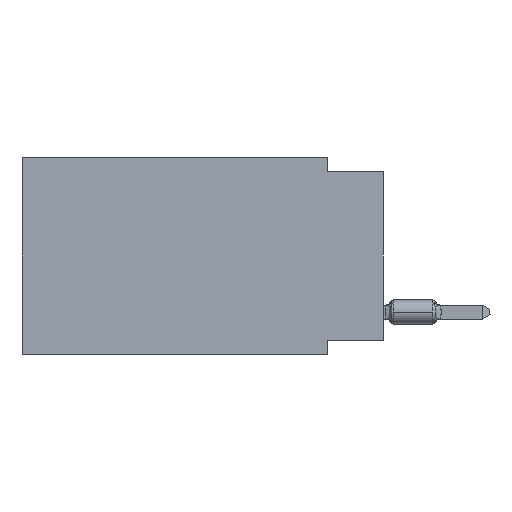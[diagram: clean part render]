
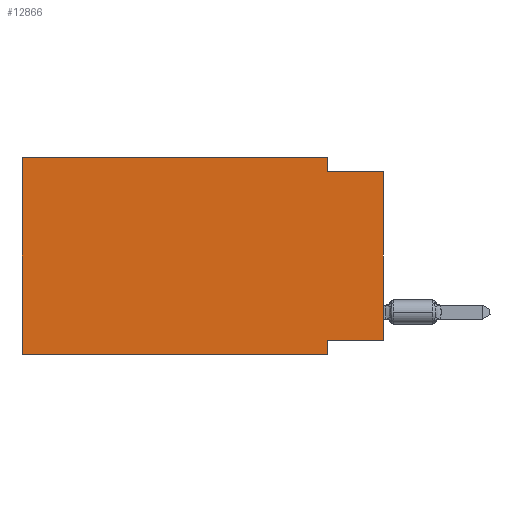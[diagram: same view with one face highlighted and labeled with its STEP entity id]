
A CAD part, left-side view. The second image highlights one B-rep face of the part: STEP entity #12866.
In plain terms, the highlighted planar face has unit normal (-1, 0, 0).
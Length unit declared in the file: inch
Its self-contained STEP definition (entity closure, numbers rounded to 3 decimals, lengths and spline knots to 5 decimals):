
#143 = EDGE_LOOP ( 'NONE', ( #57750, #5036, #26587, #40069, #41600, #67561, #18954, #63078 ) ) ;
#573 = LINE ( 'NONE', #1650, #47696 ) ;
#854 = CARTESIAN_POINT ( 'NONE',  ( 0., 0., -0.025 ) ) ;
#1492 = DIRECTION ( 'NONE',  ( 0., -1., 0. ) ) ;
#1650 = CARTESIAN_POINT ( 'NONE',  ( 0., 0., 0. ) ) ;
#2251 = VERTEX_POINT ( 'NONE', #854 ) ;
#2700 = AXIS2_PLACEMENT_3D ( 'NONE', #33103, #27999, #16654 ) ;
#3034 = EDGE_CURVE ( 'NONE', #63073, #41070, #44069, .T. ) ;
#5036 = ORIENTED_EDGE ( 'NONE', *, *, #12975, .F. ) ;
#5230 = EDGE_CURVE ( 'NONE', #29699, #2251, #573, .T. ) ;
#5494 = VERTEX_POINT ( 'NONE', #10653 ) ;
#9241 = VERTEX_POINT ( 'NONE', #39846 ) ;
#10653 = CARTESIAN_POINT ( 'NONE',  ( 0., 0.1, 0. ) ) ;
#12866 = ADVANCED_FACE ( 'NONE', ( #37851 ), #61591, .F. ) ;
#12975 = EDGE_CURVE ( 'NONE', #13869, #2251, #32755, .T. ) ;
#13869 = VERTEX_POINT ( 'NONE', #43752 ) ;
#14903 = VECTOR ( 'NONE', #70782, 39.37008 ) ;
#15004 = LINE ( 'NONE', #15367, #36095 ) ;
#15367 = CARTESIAN_POINT ( 'NONE',  ( 0., 0., -0.325 ) ) ;
#16654 = DIRECTION ( 'NONE',  ( 0., 0., -1. ) ) ;
#17293 = CARTESIAN_POINT ( 'NONE',  ( 0., 0.645, -0.35 ) ) ;
#18954 = ORIENTED_EDGE ( 'NONE', *, *, #43424, .F. ) ;
#20109 = LINE ( 'NONE', #42380, #58778 ) ;
#21126 = CARTESIAN_POINT ( 'NONE',  ( 0., 0.1, -0.35 ) ) ;
#21906 = CARTESIAN_POINT ( 'NONE',  ( 0., 0.1, -0.35 ) ) ;
#22706 = CARTESIAN_POINT ( 'NONE',  ( 0., 0.645, -0.35 ) ) ;
#26019 = VECTOR ( 'NONE', #44044, 39.37008 ) ;
#26307 = DIRECTION ( 'NONE',  ( 0., -1., 0. ) ) ;
#26587 = ORIENTED_EDGE ( 'NONE', *, *, #45945, .F. ) ;
#26660 = EDGE_CURVE ( 'NONE', #41070, #5494, #20109, .T. ) ;
#27999 = DIRECTION ( 'NONE',  ( 1., 0., 0. ) ) ;
#28007 = DIRECTION ( 'NONE',  ( 0., 0., 1. ) ) ;
#29699 = VERTEX_POINT ( 'NONE', #39610 ) ;
#32711 = EDGE_CURVE ( 'NONE', #29699, #9241, #15004, .T. ) ;
#32755 = LINE ( 'NONE', #55020, #26019 ) ;
#33103 = CARTESIAN_POINT ( 'NONE',  ( 0., 0.645, 0. ) ) ;
#33259 = DIRECTION ( 'NONE',  ( 0., 0., -1. ) ) ;
#36095 = VECTOR ( 'NONE', #47892, 39.37008 ) ;
#37851 = FACE_OUTER_BOUND ( 'NONE', #143, .T. ) ;
#39610 = CARTESIAN_POINT ( 'NONE',  ( 0., 0., -0.325 ) ) ;
#39846 = CARTESIAN_POINT ( 'NONE',  ( 0., 0.1, -0.325 ) ) ;
#40069 = ORIENTED_EDGE ( 'NONE', *, *, #26660, .F. ) ;
#40533 = LINE ( 'NONE', #62452, #57853 ) ;
#41070 = VERTEX_POINT ( 'NONE', #47830 ) ;
#41600 = ORIENTED_EDGE ( 'NONE', *, *, #3034, .F. ) ;
#42380 = CARTESIAN_POINT ( 'NONE',  ( 0., 0.645, 0. ) ) ;
#43424 = EDGE_CURVE ( 'NONE', #9241, #46297, #48925, .T. ) ;
#43752 = CARTESIAN_POINT ( 'NONE',  ( 0., 0.1, -0.025 ) ) ;
#43954 = VECTOR ( 'NONE', #1492, 39.37008 ) ;
#44044 = DIRECTION ( 'NONE',  ( 0., -1., 0. ) ) ;
#44069 = LINE ( 'NONE', #60894, #14903 ) ;
#44167 = DIRECTION ( 'NONE',  ( 0., 0., -1. ) ) ;
#45945 = EDGE_CURVE ( 'NONE', #5494, #13869, #40533, .T. ) ;
#46297 = VERTEX_POINT ( 'NONE', #21126 ) ;
#47696 = VECTOR ( 'NONE', #28007, 39.37008 ) ;
#47830 = CARTESIAN_POINT ( 'NONE',  ( 0., 0.645, 0. ) ) ;
#47892 = DIRECTION ( 'NONE',  ( 0., 1., 0. ) ) ;
#48925 = LINE ( 'NONE', #21906, #71616 ) ;
#51552 = LINE ( 'NONE', #22706, #43954 ) ;
#55020 = CARTESIAN_POINT ( 'NONE',  ( 0., 0., -0.025 ) ) ;
#57750 = ORIENTED_EDGE ( 'NONE', *, *, #5230, .T. ) ;
#57853 = VECTOR ( 'NONE', #33259, 39.37008 ) ;
#58778 = VECTOR ( 'NONE', #26307, 39.37008 ) ;
#60894 = CARTESIAN_POINT ( 'NONE',  ( 0., 0.645, 0. ) ) ;
#61591 = PLANE ( 'NONE',  #2700 ) ;
#62452 = CARTESIAN_POINT ( 'NONE',  ( 0., 0.1, 0. ) ) ;
#63073 = VERTEX_POINT ( 'NONE', #17293 ) ;
#63078 = ORIENTED_EDGE ( 'NONE', *, *, #32711, .F. ) ;
#64379 = EDGE_CURVE ( 'NONE', #63073, #46297, #51552, .T. ) ;
#67561 = ORIENTED_EDGE ( 'NONE', *, *, #64379, .T. ) ;
#70782 = DIRECTION ( 'NONE',  ( 0., 0., 1. ) ) ;
#71616 = VECTOR ( 'NONE', #44167, 39.37008 ) ;
